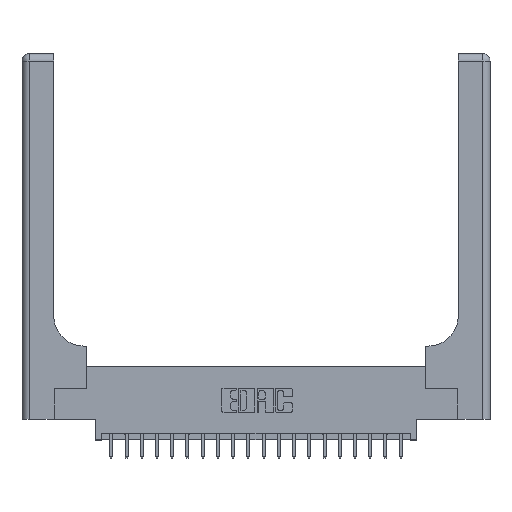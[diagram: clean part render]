
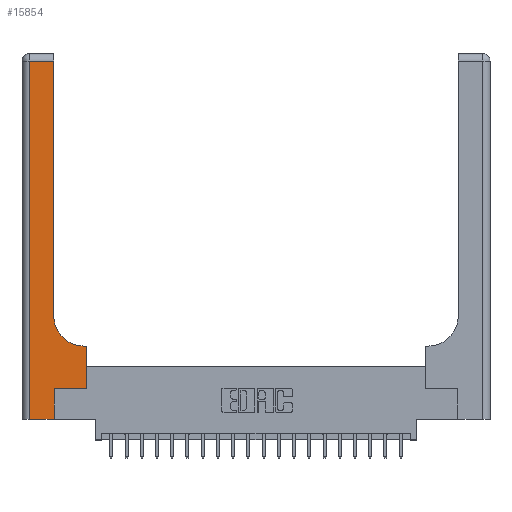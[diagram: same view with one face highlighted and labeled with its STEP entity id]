
A CAD part, top view. The second image highlights one B-rep face of the part: STEP entity #15854.
In plain terms, the highlighted planar face has unit normal (0, 0, 1).
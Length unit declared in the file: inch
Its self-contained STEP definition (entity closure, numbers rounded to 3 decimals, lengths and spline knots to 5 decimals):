
#1 = ORIENTED_EDGE ( 'NONE', *, *, #245, .T. ) ;
#21 = VECTOR ( 'NONE', #4080, 39.37008 ) ;
#64 = FACE_OUTER_BOUND ( 'NONE', #17880, .T. ) ;
#245 = EDGE_CURVE ( 'NONE', #5270, #14212, #13327, .T. ) ;
#261 = LINE ( 'NONE', #1024, #8624 ) ;
#435 = DIRECTION ( 'NONE',  ( 0., 1., 0. ) ) ;
#887 = ORIENTED_EDGE ( 'NONE', *, *, #15851, .T. ) ;
#959 = DIRECTION ( 'NONE',  ( 0., 0., -1. ) ) ;
#1024 = CARTESIAN_POINT ( 'NONE',  ( 0., 0., 0.37 ) ) ;
#2119 = ORIENTED_EDGE ( 'NONE', *, *, #15026, .T. ) ;
#2565 = EDGE_CURVE ( 'NONE', #21215, #10530, #19856, .T. ) ;
#2667 = DIRECTION ( 'NONE',  ( 0., 0., -1. ) ) ;
#2730 = DIRECTION ( 'NONE',  ( 1., 0., 0. ) ) ;
#2861 = VECTOR ( 'NONE', #8875, 39.37008 ) ;
#3487 = DIRECTION ( 'NONE',  ( 0., -1., 0. ) ) ;
#3661 = ORIENTED_EDGE ( 'NONE', *, *, #2565, .T. ) ;
#3716 = CARTESIAN_POINT ( 'NONE',  ( 0., 2.94, 0.37 ) ) ;
#4080 = DIRECTION ( 'NONE',  ( -1., 0., 0. ) ) ;
#4541 = CIRCLE ( 'NONE', #13419, 0.25 ) ;
#4823 = DIRECTION ( 'NONE',  ( 0., 1., 0. ) ) ;
#5270 = VERTEX_POINT ( 'NONE', #17251 ) ;
#5741 = LINE ( 'NONE', #10454, #15072 ) ;
#6071 = ORIENTED_EDGE ( 'NONE', *, *, #11837, .T. ) ;
#6296 = CARTESIAN_POINT ( 'NONE',  ( 0.528, 0.25, 0.37 ) ) ;
#6481 = CARTESIAN_POINT ( 'NONE',  ( 0.51, 0.6, 0.37 ) ) ;
#6819 = CARTESIAN_POINT ( 'NONE',  ( 0.06, 3., 0.37 ) ) ;
#6865 = LINE ( 'NONE', #14752, #15674 ) ;
#7127 = CARTESIAN_POINT ( 'NONE',  ( 0.26, 0.6, 0.37 ) ) ;
#7416 = VECTOR ( 'NONE', #20251, 39.37008 ) ;
#7599 = CARTESIAN_POINT ( 'NONE',  ( 0., 3., 0.37 ) ) ;
#7751 = CARTESIAN_POINT ( 'NONE',  ( 0.06, 2.94, 0.37 ) ) ;
#8134 = LINE ( 'NONE', #6819, #20157 ) ;
#8383 = VERTEX_POINT ( 'NONE', #11555 ) ;
#8624 = VECTOR ( 'NONE', #2730, 39.37008 ) ;
#8875 = DIRECTION ( 'NONE',  ( 0., 1., 0. ) ) ;
#9064 = VERTEX_POINT ( 'NONE', #19915 ) ;
#9318 = ORIENTED_EDGE ( 'NONE', *, *, #17420, .T. ) ;
#9687 = ORIENTED_EDGE ( 'NONE', *, *, #15415, .T. ) ;
#9795 = EDGE_CURVE ( 'NONE', #14212, #21301, #8134, .T. ) ;
#10368 = ORIENTED_EDGE ( 'NONE', *, *, #15062, .T. ) ;
#10454 = CARTESIAN_POINT ( 'NONE',  ( 0.26, 3., 0.37 ) ) ;
#10530 = VERTEX_POINT ( 'NONE', #16722 ) ;
#10576 = CARTESIAN_POINT ( 'NONE',  ( 0.265, 0.25, 0.37 ) ) ;
#10992 = CARTESIAN_POINT ( 'NONE',  ( 0.51, 0.85, 0.37 ) ) ;
#11349 = LINE ( 'NONE', #10576, #15693 ) ;
#11546 = VERTEX_POINT ( 'NONE', #6296 ) ;
#11555 = CARTESIAN_POINT ( 'NONE',  ( 0.528, 0.6, 0.37 ) ) ;
#11837 = EDGE_CURVE ( 'NONE', #9064, #5270, #5741, .T. ) ;
#12298 = VERTEX_POINT ( 'NONE', #6481 ) ;
#12604 = DIRECTION ( 'NONE',  ( 1., 0., 0. ) ) ;
#12726 = CARTESIAN_POINT ( 'NONE',  ( 0.265, 0., 0.37 ) ) ;
#13327 = LINE ( 'NONE', #3716, #21 ) ;
#13419 = AXIS2_PLACEMENT_3D ( 'NONE', #10992, #959, #12604 ) ;
#14212 = VERTEX_POINT ( 'NONE', #7751 ) ;
#14223 = PLANE ( 'NONE',  #17765 ) ;
#14296 = DIRECTION ( 'NONE',  ( -1., 0., 0. ) ) ;
#14752 = CARTESIAN_POINT ( 'NONE',  ( 0.528, 0.25, 0.37 ) ) ;
#15026 = EDGE_CURVE ( 'NONE', #8383, #12298, #21002, .T. ) ;
#15062 = EDGE_CURVE ( 'NONE', #10530, #11546, #11349, .T. ) ;
#15072 = VECTOR ( 'NONE', #435, 39.37008 ) ;
#15415 = EDGE_CURVE ( 'NONE', #11546, #8383, #6865, .T. ) ;
#15456 = DIRECTION ( 'NONE',  ( 1., 0., 0. ) ) ;
#15674 = VECTOR ( 'NONE', #4823, 39.37008 ) ;
#15693 = VECTOR ( 'NONE', #15456, 39.37008 ) ;
#15851 = EDGE_CURVE ( 'NONE', #12298, #9064, #4541, .T. ) ;
#15854 = ADVANCED_FACE ( 'NONE', ( #64 ), #14223, .F. ) ;
#16056 = ORIENTED_EDGE ( 'NONE', *, *, #9795, .T. ) ;
#16722 = CARTESIAN_POINT ( 'NONE',  ( 0.265, 0.25, 0.37 ) ) ;
#17059 = CARTESIAN_POINT ( 'NONE',  ( 0.265, 0., 0.37 ) ) ;
#17251 = CARTESIAN_POINT ( 'NONE',  ( 0.26, 2.94, 0.37 ) ) ;
#17420 = EDGE_CURVE ( 'NONE', #21301, #21215, #261, .T. ) ;
#17765 = AXIS2_PLACEMENT_3D ( 'NONE', #7599, #2667, #14296 ) ;
#17880 = EDGE_LOOP ( 'NONE', ( #6071, #1, #16056, #9318, #3661, #10368, #9687, #2119, #887 ) ) ;
#19418 = CARTESIAN_POINT ( 'NONE',  ( 0.06, 0., 0.37 ) ) ;
#19856 = LINE ( 'NONE', #17059, #2861 ) ;
#19915 = CARTESIAN_POINT ( 'NONE',  ( 0.26, 0.85, 0.37 ) ) ;
#20157 = VECTOR ( 'NONE', #3487, 39.37008 ) ;
#20251 = DIRECTION ( 'NONE',  ( -1., 0., 0. ) ) ;
#21002 = LINE ( 'NONE', #7127, #7416 ) ;
#21215 = VERTEX_POINT ( 'NONE', #12726 ) ;
#21301 = VERTEX_POINT ( 'NONE', #19418 ) ;
